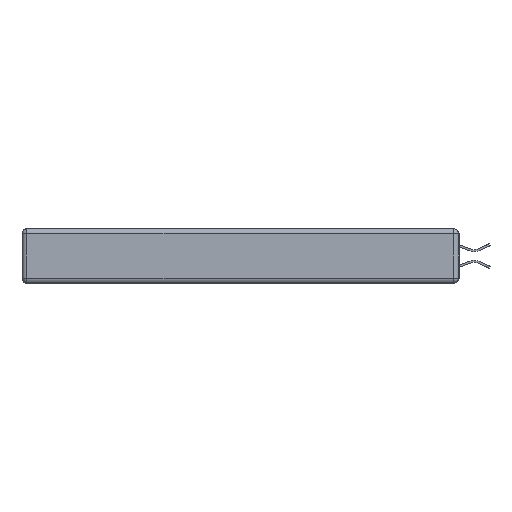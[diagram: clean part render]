
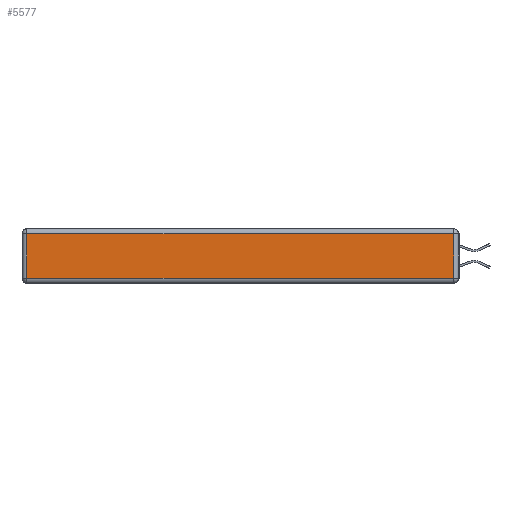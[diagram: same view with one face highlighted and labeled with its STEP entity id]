
A CAD part, left-side view. The second image highlights one B-rep face of the part: STEP entity #5577.
In plain terms, the highlighted planar face has unit normal (-1, 0, 0).
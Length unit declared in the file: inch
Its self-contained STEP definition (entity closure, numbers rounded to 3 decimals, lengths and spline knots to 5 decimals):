
#3375 = CARTESIAN_POINT ( 'NONE',  ( 0., 0.03, -0.313 ) ) ;
#4465 = VERTEX_POINT ( 'NONE', #28094 ) ;
#4748 = EDGE_CURVE ( 'NONE', #27354, #12774, #25606, .T. ) ;
#4988 = CARTESIAN_POINT ( 'NONE',  ( 0., 0., -0.343 ) ) ;
#5128 = LINE ( 'NONE', #23642, #11189 ) ;
#5266 = CARTESIAN_POINT ( 'NONE',  ( 0., 2.72, -0.343 ) ) ;
#5577 = ADVANCED_FACE ( 'NONE', ( #26735 ), #19366, .T. ) ;
#5622 = VECTOR ( 'NONE', #19644, 39.37008 ) ;
#5703 = CARTESIAN_POINT ( 'NONE',  ( 0., 2.72, -0.313 ) ) ;
#6183 = DIRECTION ( 'NONE',  ( 0., -1., 0. ) ) ;
#6660 = VERTEX_POINT ( 'NONE', #5703 ) ;
#8734 = EDGE_CURVE ( 'NONE', #4465, #6660, #18031, .T. ) ;
#9258 = DIRECTION ( 'NONE',  ( 0., 1., 0. ) ) ;
#11189 = VECTOR ( 'NONE', #9258, 39.37008 ) ;
#12242 = DIRECTION ( 'NONE',  ( -1., 0., 0. ) ) ;
#12774 = VERTEX_POINT ( 'NONE', #17122 ) ;
#12791 = VECTOR ( 'NONE', #30808, 39.37008 ) ;
#13492 = AXIS2_PLACEMENT_3D ( 'NONE', #4988, #12242, #17090 ) ;
#17090 = DIRECTION ( 'NONE',  ( 0., 0., 1. ) ) ;
#17122 = CARTESIAN_POINT ( 'NONE',  ( 0., 0.03, -0.03 ) ) ;
#18031 = LINE ( 'NONE', #5266, #5622 ) ;
#19060 = VECTOR ( 'NONE', #6183, 39.37008 ) ;
#19366 = PLANE ( 'NONE',  #13492 ) ;
#19644 = DIRECTION ( 'NONE',  ( 0., 0., -1. ) ) ;
#19729 = ORIENTED_EDGE ( 'NONE', *, *, #4748, .T. ) ;
#20757 = ORIENTED_EDGE ( 'NONE', *, *, #25513, .T. ) ;
#22060 = LINE ( 'NONE', #22195, #19060 ) ;
#22186 = EDGE_CURVE ( 'NONE', #12774, #4465, #5128, .T. ) ;
#22195 = CARTESIAN_POINT ( 'NONE',  ( 0., 0., -0.313 ) ) ;
#23186 = EDGE_LOOP ( 'NONE', ( #20757, #19729, #26724, #23914 ) ) ;
#23642 = CARTESIAN_POINT ( 'NONE',  ( 0., 2.75, -0.03 ) ) ;
#23914 = ORIENTED_EDGE ( 'NONE', *, *, #8734, .T. ) ;
#25513 = EDGE_CURVE ( 'NONE', #6660, #27354, #22060, .T. ) ;
#25606 = LINE ( 'NONE', #28369, #12791 ) ;
#26724 = ORIENTED_EDGE ( 'NONE', *, *, #22186, .T. ) ;
#26735 = FACE_OUTER_BOUND ( 'NONE', #23186, .T. ) ;
#27354 = VERTEX_POINT ( 'NONE', #3375 ) ;
#28094 = CARTESIAN_POINT ( 'NONE',  ( 0., 2.72, -0.03 ) ) ;
#28369 = CARTESIAN_POINT ( 'NONE',  ( 0., 0.03, -0.343 ) ) ;
#30808 = DIRECTION ( 'NONE',  ( 0., 0., 1. ) ) ;
